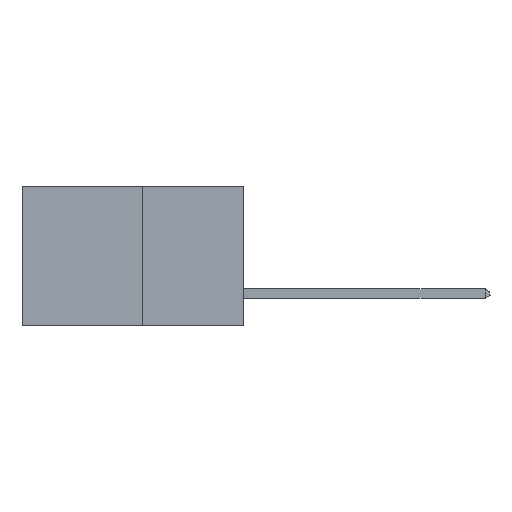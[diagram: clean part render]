
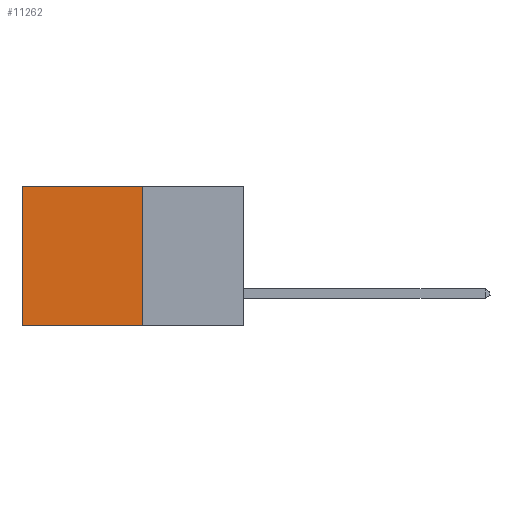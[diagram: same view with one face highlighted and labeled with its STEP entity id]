
A CAD part, left-side view. The second image highlights one B-rep face of the part: STEP entity #11262.
In plain terms, the highlighted planar face has unit normal (-1, 0, 0).
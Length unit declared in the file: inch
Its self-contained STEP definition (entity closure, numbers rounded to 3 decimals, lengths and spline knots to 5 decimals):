
#89 = CARTESIAN_POINT ( 'NONE',  ( 0.277, 0.27, -0.37 ) ) ;
#434 = VECTOR ( 'NONE', #10991, 39.37008 ) ;
#559 = DIRECTION ( 'NONE',  ( 0., 1., 0. ) ) ;
#1008 = CARTESIAN_POINT ( 'NONE',  ( 0.277, 0.27, -0.37 ) ) ;
#1242 = VECTOR ( 'NONE', #3261, 39.37008 ) ;
#1407 = VERTEX_POINT ( 'NONE', #89 ) ;
#2629 = PLANE ( 'NONE',  #7948 ) ;
#2839 = DIRECTION ( 'NONE',  ( 0., 0., -1. ) ) ;
#3018 = VERTEX_POINT ( 'NONE', #11886 ) ;
#3093 = FACE_OUTER_BOUND ( 'NONE', #5216, .T. ) ;
#3261 = DIRECTION ( 'NONE',  ( 0., 0., -1. ) ) ;
#3414 = LINE ( 'NONE', #4713, #434 ) ;
#3711 = DIRECTION ( 'NONE',  ( 1., 0., 0. ) ) ;
#3851 = ORIENTED_EDGE ( 'NONE', *, *, #9824, .T. ) ;
#3936 = CARTESIAN_POINT ( 'NONE',  ( 0.277, 0.59, -0.37 ) ) ;
#4282 = VERTEX_POINT ( 'NONE', #12325 ) ;
#4534 = CARTESIAN_POINT ( 'NONE',  ( 0.277, 0.27, 0. ) ) ;
#4713 = CARTESIAN_POINT ( 'NONE',  ( 0.277, 0.27, 0. ) ) ;
#5114 = VERTEX_POINT ( 'NONE', #4534 ) ;
#5216 = EDGE_LOOP ( 'NONE', ( #3851, #12134, #7052, #9747 ) ) ;
#5926 = EDGE_CURVE ( 'NONE', #5114, #3018, #3414, .T. ) ;
#7052 = ORIENTED_EDGE ( 'NONE', *, *, #8632, .F. ) ;
#7300 = VECTOR ( 'NONE', #559, 39.37008 ) ;
#7353 = LINE ( 'NONE', #1008, #1242 ) ;
#7614 = LINE ( 'NONE', #10085, #7300 ) ;
#7948 = AXIS2_PLACEMENT_3D ( 'NONE', #8986, #3711, #11030 ) ;
#8632 = EDGE_CURVE ( 'NONE', #5114, #1407, #7353, .T. ) ;
#8986 = CARTESIAN_POINT ( 'NONE',  ( 0.277, 0.27, -0.37 ) ) ;
#9747 = ORIENTED_EDGE ( 'NONE', *, *, #5926, .T. ) ;
#9824 = EDGE_CURVE ( 'NONE', #3018, #4282, #11013, .T. ) ;
#10085 = CARTESIAN_POINT ( 'NONE',  ( 0.277, 0.27, -0.37 ) ) ;
#10677 = VECTOR ( 'NONE', #2839, 39.37008 ) ;
#10704 = EDGE_CURVE ( 'NONE', #1407, #4282, #7614, .T. ) ;
#10991 = DIRECTION ( 'NONE',  ( 0., 1., 0. ) ) ;
#11013 = LINE ( 'NONE', #3936, #10677 ) ;
#11030 = DIRECTION ( 'NONE',  ( 0., 0., -1. ) ) ;
#11262 = ADVANCED_FACE ( 'NONE', ( #3093 ), #2629, .F. ) ;
#11886 = CARTESIAN_POINT ( 'NONE',  ( 0.277, 0.59, 0. ) ) ;
#12134 = ORIENTED_EDGE ( 'NONE', *, *, #10704, .F. ) ;
#12325 = CARTESIAN_POINT ( 'NONE',  ( 0.277, 0.59, -0.37 ) ) ;
